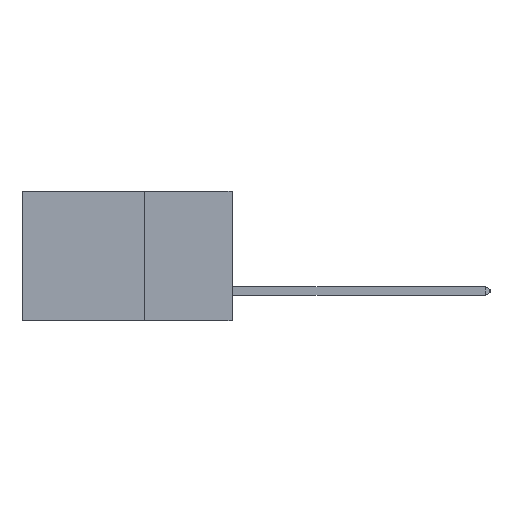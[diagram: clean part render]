
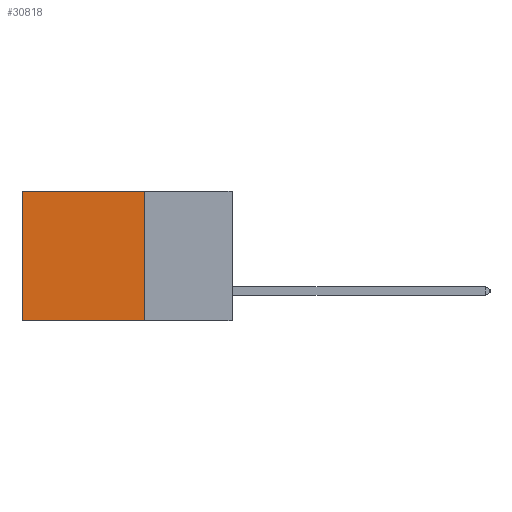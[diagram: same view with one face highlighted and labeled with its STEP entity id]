
A CAD part, left-side view. The second image highlights one B-rep face of the part: STEP entity #30818.
In plain terms, the highlighted planar face has unit normal (-1, 0, 0).
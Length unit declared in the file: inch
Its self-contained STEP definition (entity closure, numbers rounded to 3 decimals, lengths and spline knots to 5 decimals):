
#677 = LINE ( 'NONE', #18319, #7534 ) ;
#3557 = CARTESIAN_POINT ( 'NONE',  ( 0.2875, 0.25, 0. ) ) ;
#3737 = CARTESIAN_POINT ( 'NONE',  ( 0.2875, 0.25, 0. ) ) ;
#4275 = ORIENTED_EDGE ( 'NONE', *, *, #23617, .F. ) ;
#4985 = CARTESIAN_POINT ( 'NONE',  ( 0.2875, 0.25, 0. ) ) ;
#6459 = LINE ( 'NONE', #17007, #14172 ) ;
#7534 = VECTOR ( 'NONE', #21218, 39.37008 ) ;
#9441 = DIRECTION ( 'NONE',  ( 1., 0., 0. ) ) ;
#9554 = VERTEX_POINT ( 'NONE', #36137 ) ;
#10561 = CARTESIAN_POINT ( 'NONE',  ( 0.2875, 0.25, -0.37 ) ) ;
#12860 = LINE ( 'NONE', #3737, #19541 ) ;
#13420 = DIRECTION ( 'NONE',  ( 0., 1., 0. ) ) ;
#14172 = VECTOR ( 'NONE', #36931, 39.37008 ) ;
#14939 = EDGE_LOOP ( 'NONE', ( #31058, #4275, #24732, #18356 ) ) ;
#17007 = CARTESIAN_POINT ( 'NONE',  ( 0.2875, 0.6, 0. ) ) ;
#17938 = PLANE ( 'NONE',  #23853 ) ;
#18319 = CARTESIAN_POINT ( 'NONE',  ( 0.2875, 0.25, 0. ) ) ;
#18356 = ORIENTED_EDGE ( 'NONE', *, *, #24039, .T. ) ;
#18887 = VERTEX_POINT ( 'NONE', #37122 ) ;
#19032 = CARTESIAN_POINT ( 'NONE',  ( 0.2875, 0.6, -0.37 ) ) ;
#19541 = VECTOR ( 'NONE', #35337, 39.37008 ) ;
#21218 = DIRECTION ( 'NONE',  ( 0., 0., -1. ) ) ;
#21755 = VERTEX_POINT ( 'NONE', #19032 ) ;
#23617 = EDGE_CURVE ( 'NONE', #9554, #21755, #28980, .T. ) ;
#23853 = AXIS2_PLACEMENT_3D ( 'NONE', #3557, #9441, #29433 ) ;
#24039 = EDGE_CURVE ( 'NONE', #35924, #18887, #12860, .T. ) ;
#24732 = ORIENTED_EDGE ( 'NONE', *, *, #36228, .F. ) ;
#28074 = VECTOR ( 'NONE', #13420, 39.37008 ) ;
#28980 = LINE ( 'NONE', #10561, #28074 ) ;
#29433 = DIRECTION ( 'NONE',  ( 0., 0., -1. ) ) ;
#29860 = FACE_OUTER_BOUND ( 'NONE', #14939, .T. ) ;
#30818 = ADVANCED_FACE ( 'NONE', ( #29860 ), #17938, .F. ) ;
#31058 = ORIENTED_EDGE ( 'NONE', *, *, #31875, .T. ) ;
#31875 = EDGE_CURVE ( 'NONE', #18887, #21755, #6459, .T. ) ;
#35337 = DIRECTION ( 'NONE',  ( 0., 1., 0. ) ) ;
#35924 = VERTEX_POINT ( 'NONE', #4985 ) ;
#36137 = CARTESIAN_POINT ( 'NONE',  ( 0.2875, 0.25, -0.37 ) ) ;
#36228 = EDGE_CURVE ( 'NONE', #35924, #9554, #677, .T. ) ;
#36931 = DIRECTION ( 'NONE',  ( 0., 0., -1. ) ) ;
#37122 = CARTESIAN_POINT ( 'NONE',  ( 0.2875, 0.6, 0. ) ) ;
